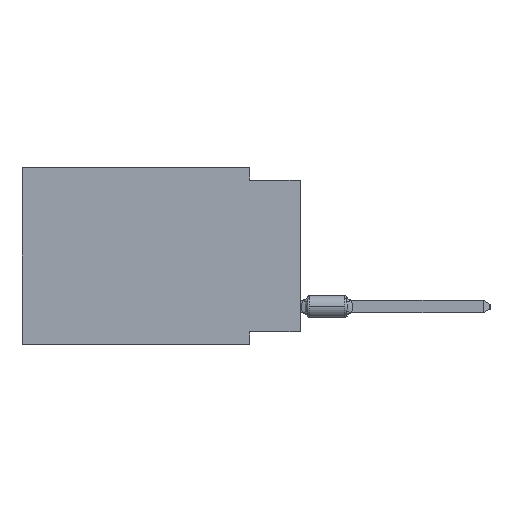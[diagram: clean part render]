
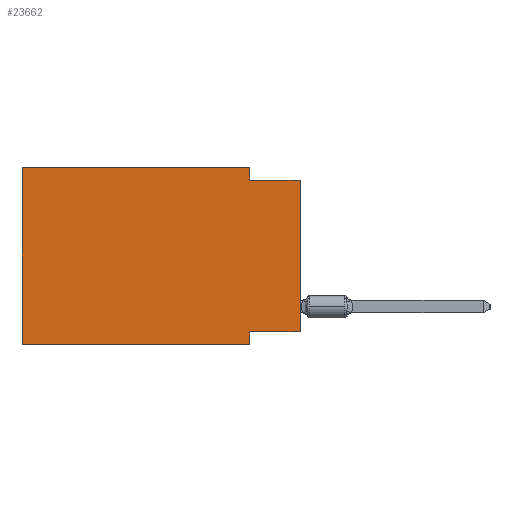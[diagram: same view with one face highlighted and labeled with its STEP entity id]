
A CAD part, left-side view. The second image highlights one B-rep face of the part: STEP entity #23662.
In plain terms, the highlighted planar face has unit normal (-1, 0, 0).
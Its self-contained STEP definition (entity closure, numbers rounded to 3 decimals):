
#2326 = LINE ( 'NONE', #86935, #26582 ) ;
#2776 = LINE ( 'NONE', #19859, #11713 ) ;
#4598 = ORIENTED_EDGE ( 'NONE', *, *, #65049, .F. ) ;
#5145 = ORIENTED_EDGE ( 'NONE', *, *, #76521, .T. ) ;
#5191 = VERTEX_POINT ( 'NONE', #83332 ) ;
#5258 = VERTEX_POINT ( 'NONE', #24357 ) ;
#11699 = CARTESIAN_POINT ( 'NONE',  ( 0., 2.54, -8.89 ) ) ;
#11713 = VECTOR ( 'NONE', #88365, 1000. ) ;
#11842 = CARTESIAN_POINT ( 'NONE',  ( 0., 0., -0.635 ) ) ;
#12682 = CARTESIAN_POINT ( 'NONE',  ( 0., 2.54, 0. ) ) ;
#15201 = PLANE ( 'NONE',  #69441 ) ;
#15438 = EDGE_LOOP ( 'NONE', ( #25818, #93333, #39916, #4598, #89479, #5145, #22406, #25407 ) ) ;
#18026 = CARTESIAN_POINT ( 'NONE',  ( 0., 0., -8.255 ) ) ;
#18324 = VERTEX_POINT ( 'NONE', #30801 ) ;
#19859 = CARTESIAN_POINT ( 'NONE',  ( 0., 0., 0. ) ) ;
#21515 = CARTESIAN_POINT ( 'NONE',  ( 0., 0., -8.255 ) ) ;
#22406 = ORIENTED_EDGE ( 'NONE', *, *, #39984, .F. ) ;
#23662 = ADVANCED_FACE ( 'NONE', ( #53001 ), #15201, .F. ) ;
#24357 = CARTESIAN_POINT ( 'NONE',  ( 0., 2.54, -8.89 ) ) ;
#25407 = ORIENTED_EDGE ( 'NONE', *, *, #40773, .F. ) ;
#25818 = ORIENTED_EDGE ( 'NONE', *, *, #54664, .T. ) ;
#26042 = DIRECTION ( 'NONE',  ( 0., 0., 1. ) ) ;
#26582 = VECTOR ( 'NONE', #95489, 1000. ) ;
#30801 = CARTESIAN_POINT ( 'NONE',  ( 0., 2.54, -0.635 ) ) ;
#30875 = LINE ( 'NONE', #61619, #88784 ) ;
#34473 = VECTOR ( 'NONE', #83062, 1000. ) ;
#37713 = VECTOR ( 'NONE', #57315, 1000. ) ;
#39916 = ORIENTED_EDGE ( 'NONE', *, *, #78052, .F. ) ;
#39984 = EDGE_CURVE ( 'NONE', #42554, #5258, #43420, .T. ) ;
#40435 = EDGE_CURVE ( 'NONE', #18324, #80414, #75031, .T. ) ;
#40773 = EDGE_CURVE ( 'NONE', #57747, #42554, #81458, .T. ) ;
#42554 = VERTEX_POINT ( 'NONE', #50863 ) ;
#42903 = LINE ( 'NONE', #12682, #65346 ) ;
#43420 = LINE ( 'NONE', #11699, #50736 ) ;
#44955 = CARTESIAN_POINT ( 'NONE',  ( 0., 13.97, 0. ) ) ;
#49218 = LINE ( 'NONE', #88970, #52794 ) ;
#50736 = VECTOR ( 'NONE', #74176, 1000. ) ;
#50863 = CARTESIAN_POINT ( 'NONE',  ( 0., 2.54, -8.255 ) ) ;
#52794 = VECTOR ( 'NONE', #26042, 1000. ) ;
#53001 = FACE_OUTER_BOUND ( 'NONE', #15438, .T. ) ;
#53041 = VERTEX_POINT ( 'NONE', #81705 ) ;
#54664 = EDGE_CURVE ( 'NONE', #57747, #80414, #2776, .T. ) ;
#57315 = DIRECTION ( 'NONE',  ( 0., 1., 0. ) ) ;
#57747 = VERTEX_POINT ( 'NONE', #21515 ) ;
#61619 = CARTESIAN_POINT ( 'NONE',  ( 0., 13.97, 0. ) ) ;
#62050 = DIRECTION ( 'NONE',  ( 0., 0., -1. ) ) ;
#64622 = CARTESIAN_POINT ( 'NONE',  ( 0., 2.54, 0. ) ) ;
#65049 = EDGE_CURVE ( 'NONE', #5191, #77832, #30875, .T. ) ;
#65346 = VECTOR ( 'NONE', #97306, 1000. ) ;
#69441 = AXIS2_PLACEMENT_3D ( 'NONE', #44955, #83721, #62050 ) ;
#74176 = DIRECTION ( 'NONE',  ( 0., 0., -1. ) ) ;
#75031 = LINE ( 'NONE', #90639, #34473 ) ;
#76521 = EDGE_CURVE ( 'NONE', #53041, #5258, #2326, .T. ) ;
#77832 = VERTEX_POINT ( 'NONE', #64622 ) ;
#78052 = EDGE_CURVE ( 'NONE', #77832, #18324, #42903, .T. ) ;
#80414 = VERTEX_POINT ( 'NONE', #11842 ) ;
#81458 = LINE ( 'NONE', #18026, #37713 ) ;
#81705 = CARTESIAN_POINT ( 'NONE',  ( 0., 13.97, -8.89 ) ) ;
#83062 = DIRECTION ( 'NONE',  ( 0., -1., 0. ) ) ;
#83332 = CARTESIAN_POINT ( 'NONE',  ( 0., 13.97, 0. ) ) ;
#83721 = DIRECTION ( 'NONE',  ( 1., 0., 0. ) ) ;
#86935 = CARTESIAN_POINT ( 'NONE',  ( 0., 13.97, -8.89 ) ) ;
#88365 = DIRECTION ( 'NONE',  ( 0., 0., 1. ) ) ;
#88784 = VECTOR ( 'NONE', #99393, 1000. ) ;
#88970 = CARTESIAN_POINT ( 'NONE',  ( 0., 13.97, 0. ) ) ;
#89479 = ORIENTED_EDGE ( 'NONE', *, *, #90713, .F. ) ;
#90639 = CARTESIAN_POINT ( 'NONE',  ( 0., 0., -0.635 ) ) ;
#90713 = EDGE_CURVE ( 'NONE', #53041, #5191, #49218, .T. ) ;
#93333 = ORIENTED_EDGE ( 'NONE', *, *, #40435, .F. ) ;
#95489 = DIRECTION ( 'NONE',  ( 0., -1., 0. ) ) ;
#97306 = DIRECTION ( 'NONE',  ( 0., 0., -1. ) ) ;
#99393 = DIRECTION ( 'NONE',  ( 0., -1., 0. ) ) ;
